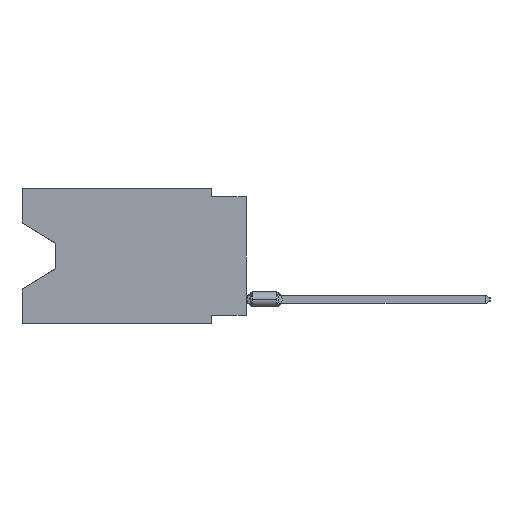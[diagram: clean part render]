
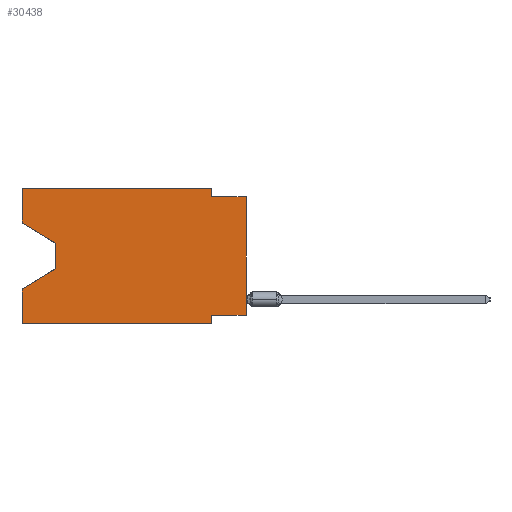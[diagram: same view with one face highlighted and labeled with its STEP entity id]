
A CAD part, left-side view. The second image highlights one B-rep face of the part: STEP entity #30438.
In plain terms, the highlighted planar face has unit normal (-1, 0, 0).
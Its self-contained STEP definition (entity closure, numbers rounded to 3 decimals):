
#1979 = LINE ( 'NONE', #43179, #77776 ) ;
#4588 = LINE ( 'NONE', #56819, #46609 ) ;
#4597 = ORIENTED_EDGE ( 'NONE', *, *, #36940, .T. ) ;
#5517 = AXIS2_PLACEMENT_3D ( 'NONE', #82453, #75874, #85919 ) ;
#5862 = EDGE_CURVE ( 'NONE', #33612, #69223, #4588, .T. ) ;
#5935 = VERTEX_POINT ( 'NONE', #73424 ) ;
#6325 = ORIENTED_EDGE ( 'NONE', *, *, #48691, .T. ) ;
#7240 = DIRECTION ( 'NONE',  ( 0., -1., 0. ) ) ;
#7904 = VERTEX_POINT ( 'NONE', #71953 ) ;
#8306 = VECTOR ( 'NONE', #29254, 1000. ) ;
#8426 = EDGE_CURVE ( 'NONE', #27700, #70410, #68602, .T. ) ;
#8481 = CARTESIAN_POINT ( 'NONE',  ( 0., 16.383, 0. ) ) ;
#8926 = VERTEX_POINT ( 'NONE', #12883 ) ;
#9982 = ORIENTED_EDGE ( 'NONE', *, *, #63678, .F. ) ;
#11983 = CARTESIAN_POINT ( 'NONE',  ( 0., 13.97, -4.013 ) ) ;
#12337 = LINE ( 'NONE', #18046, #13202 ) ;
#12883 = CARTESIAN_POINT ( 'NONE',  ( 0., 0., -9.271 ) ) ;
#13202 = VECTOR ( 'NONE', #44823, 1000. ) ;
#14134 = LINE ( 'NONE', #75090, #79700 ) ;
#14485 = VECTOR ( 'NONE', #7240, 1000. ) ;
#15439 = VECTOR ( 'NONE', #64094, 1000. ) ;
#16040 = DIRECTION ( 'NONE',  ( 0., -1., 0. ) ) ;
#17348 = VECTOR ( 'NONE', #86128, 1000. ) ;
#18046 = CARTESIAN_POINT ( 'NONE',  ( 0., 2.54, 0. ) ) ;
#18390 = VERTEX_POINT ( 'NONE', #29058 ) ;
#18963 = VECTOR ( 'NONE', #73082, 1000. ) ;
#20231 = CARTESIAN_POINT ( 'NONE',  ( 0., 2.54, -0.635 ) ) ;
#20592 = CARTESIAN_POINT ( 'NONE',  ( 0., 16.383, 0. ) ) ;
#25539 = ORIENTED_EDGE ( 'NONE', *, *, #38666, .F. ) ;
#25931 = VECTOR ( 'NONE', #35241, 1000. ) ;
#26646 = ORIENTED_EDGE ( 'NONE', *, *, #86237, .T. ) ;
#27700 = VERTEX_POINT ( 'NONE', #74580 ) ;
#28517 = VERTEX_POINT ( 'NONE', #54055 ) ;
#28533 = VECTOR ( 'NONE', #47363, 1000. ) ;
#28922 = PLANE ( 'NONE',  #5517 ) ;
#29028 = DIRECTION ( 'NONE',  ( 0., 0., 1. ) ) ;
#29058 = CARTESIAN_POINT ( 'NONE',  ( 0., 0., -0.635 ) ) ;
#29254 = DIRECTION ( 'NONE',  ( 0., 1., 0. ) ) ;
#30438 = ADVANCED_FACE ( 'NONE', ( #35499 ), #28922, .F. ) ;
#33612 = VERTEX_POINT ( 'NONE', #84687 ) ;
#33879 = ORIENTED_EDGE ( 'NONE', *, *, #54874, .F. ) ;
#35241 = DIRECTION ( 'NONE',  ( 0., 0., 1. ) ) ;
#35499 = FACE_OUTER_BOUND ( 'NONE', #43197, .T. ) ;
#35676 = ORIENTED_EDGE ( 'NONE', *, *, #65552, .F. ) ;
#36940 = EDGE_CURVE ( 'NONE', #8926, #18390, #14134, .T. ) ;
#38113 = CARTESIAN_POINT ( 'NONE',  ( 0., 13.97, -4.013 ) ) ;
#38666 = EDGE_CURVE ( 'NONE', #73245, #5935, #69809, .T. ) ;
#40953 = ORIENTED_EDGE ( 'NONE', *, *, #69665, .F. ) ;
#41818 = VERTEX_POINT ( 'NONE', #61722 ) ;
#43179 = CARTESIAN_POINT ( 'NONE',  ( 0., 13.97, -5.893 ) ) ;
#43197 = EDGE_LOOP ( 'NONE', ( #70648, #26646, #6325, #73374, #43492, #25539, #40953, #4597, #35676, #33879, #54883, #9982 ) ) ;
#43492 = ORIENTED_EDGE ( 'NONE', *, *, #76899, .T. ) ;
#44823 = DIRECTION ( 'NONE',  ( 0., 0., -1. ) ) ;
#46533 = EDGE_CURVE ( 'NONE', #7904, #28517, #49418, .T. ) ;
#46609 = VECTOR ( 'NONE', #76980, 1000. ) ;
#47363 = DIRECTION ( 'NONE',  ( 0., 0., 1. ) ) ;
#47795 = LINE ( 'NONE', #20592, #28533 ) ;
#48691 = EDGE_CURVE ( 'NONE', #41818, #70410, #1979, .T. ) ;
#49418 = LINE ( 'NONE', #76167, #85635 ) ;
#51951 = CARTESIAN_POINT ( 'NONE',  ( 0., 0., -9.271 ) ) ;
#54055 = CARTESIAN_POINT ( 'NONE',  ( 0., 2.54, 0. ) ) ;
#54874 = EDGE_CURVE ( 'NONE', #28517, #73169, #12337, .T. ) ;
#54883 = ORIENTED_EDGE ( 'NONE', *, *, #46533, .F. ) ;
#56819 = CARTESIAN_POINT ( 'NONE',  ( 0., 16.383, -2.546 ) ) ;
#59374 = LINE ( 'NONE', #11983, #17348 ) ;
#60352 = CARTESIAN_POINT ( 'NONE',  ( 0., 0., -0.635 ) ) ;
#61722 = CARTESIAN_POINT ( 'NONE',  ( 0., 13.97, -5.893 ) ) ;
#63678 = EDGE_CURVE ( 'NONE', #33612, #7904, #47795, .T. ) ;
#64094 = DIRECTION ( 'NONE',  ( 0., 0., -1. ) ) ;
#64478 = CARTESIAN_POINT ( 'NONE',  ( 0., 16.383, -7.36 ) ) ;
#65552 = EDGE_CURVE ( 'NONE', #73169, #18390, #66920, .T. ) ;
#66920 = LINE ( 'NONE', #60352, #18963 ) ;
#68602 = LINE ( 'NONE', #8481, #25931 ) ;
#69223 = VERTEX_POINT ( 'NONE', #38113 ) ;
#69665 = EDGE_CURVE ( 'NONE', #8926, #73245, #70057, .T. ) ;
#69809 = LINE ( 'NONE', #71114, #15439 ) ;
#70057 = LINE ( 'NONE', #51951, #8306 ) ;
#70410 = VERTEX_POINT ( 'NONE', #64478 ) ;
#70648 = ORIENTED_EDGE ( 'NONE', *, *, #5862, .T. ) ;
#71114 = CARTESIAN_POINT ( 'NONE',  ( 0., 2.54, -9.906 ) ) ;
#71953 = CARTESIAN_POINT ( 'NONE',  ( 0., 16.383, 0. ) ) ;
#73082 = DIRECTION ( 'NONE',  ( 0., -1., 0. ) ) ;
#73169 = VERTEX_POINT ( 'NONE', #20231 ) ;
#73245 = VERTEX_POINT ( 'NONE', #74619 ) ;
#73374 = ORIENTED_EDGE ( 'NONE', *, *, #8426, .F. ) ;
#73424 = CARTESIAN_POINT ( 'NONE',  ( 0., 2.54, -9.906 ) ) ;
#74364 = LINE ( 'NONE', #81804, #14485 ) ;
#74580 = CARTESIAN_POINT ( 'NONE',  ( 0., 16.383, -9.906 ) ) ;
#74619 = CARTESIAN_POINT ( 'NONE',  ( 0., 2.54, -9.271 ) ) ;
#75090 = CARTESIAN_POINT ( 'NONE',  ( 0., 0., 0. ) ) ;
#75874 = DIRECTION ( 'NONE',  ( 1., 0., 0. ) ) ;
#76167 = CARTESIAN_POINT ( 'NONE',  ( 0., 16.383, 0. ) ) ;
#76899 = EDGE_CURVE ( 'NONE', #27700, #5935, #74364, .T. ) ;
#76980 = DIRECTION ( 'NONE',  ( 0., -0.855, -0.519 ) ) ;
#77776 = VECTOR ( 'NONE', #82257, 1000. ) ;
#79700 = VECTOR ( 'NONE', #29028, 1000. ) ;
#81804 = CARTESIAN_POINT ( 'NONE',  ( 0., 16.383, -9.906 ) ) ;
#82257 = DIRECTION ( 'NONE',  ( 0., 0.855, -0.519 ) ) ;
#82453 = CARTESIAN_POINT ( 'NONE',  ( 0., 16.383, 0. ) ) ;
#84687 = CARTESIAN_POINT ( 'NONE',  ( 0., 16.383, -2.546 ) ) ;
#85635 = VECTOR ( 'NONE', #16040, 1000. ) ;
#85919 = DIRECTION ( 'NONE',  ( 0., 0., -1. ) ) ;
#86128 = DIRECTION ( 'NONE',  ( 0., 0., -1. ) ) ;
#86237 = EDGE_CURVE ( 'NONE', #69223, #41818, #59374, .T. ) ;
